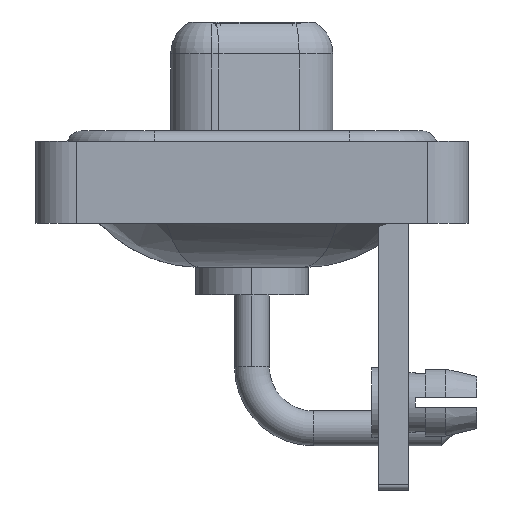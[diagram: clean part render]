
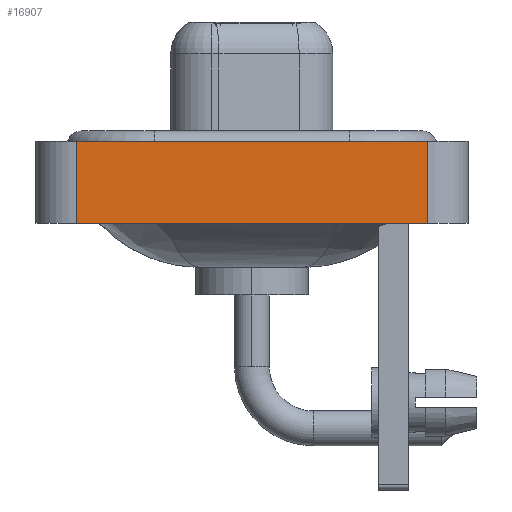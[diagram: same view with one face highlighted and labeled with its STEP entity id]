
A CAD part, left-side view. The second image highlights one B-rep face of the part: STEP entity #16907.
In plain terms, the highlighted planar face has unit normal (-1, 0, 0).
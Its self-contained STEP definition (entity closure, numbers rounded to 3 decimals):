
#25 = EDGE_CURVE ( 'NONE', #10821, #4628, #16702, .T. ) ;
#281 = LINE ( 'NONE', #15452, #17291 ) ;
#883 = VERTEX_POINT ( 'NONE', #17997 ) ;
#1345 = CARTESIAN_POINT ( 'NONE',  ( -7.25, -8.55, -3.6 ) ) ;
#1380 = ORIENTED_EDGE ( 'NONE', *, *, #2059, .F. ) ;
#1501 = CARTESIAN_POINT ( 'NONE',  ( -7.25, -8.55, 0.4 ) ) ;
#1527 = AXIS2_PLACEMENT_3D ( 'NONE', #9806, #12780, #12963 ) ;
#1547 = EDGE_CURVE ( 'NONE', #9805, #10821, #13896, .T. ) ;
#2059 = EDGE_CURVE ( 'NONE', #883, #4628, #7093, .T. ) ;
#2160 = EDGE_LOOP ( 'NONE', ( #3265, #1380, #16736, #16209 ) ) ;
#2559 = CARTESIAN_POINT ( 'NONE',  ( -7.25, -8.55, -3.6 ) ) ;
#3213 = CARTESIAN_POINT ( 'NONE',  ( -7.25, -8.55, 0.4 ) ) ;
#3265 = ORIENTED_EDGE ( 'NONE', *, *, #25, .T. ) ;
#3980 = VECTOR ( 'NONE', #8438, 1000. ) ;
#4022 = CARTESIAN_POINT ( 'NONE',  ( -7.25, -8.55, -3.6 ) ) ;
#4605 = DIRECTION ( 'NONE',  ( 0., -1., 0. ) ) ;
#4628 = VERTEX_POINT ( 'NONE', #1501 ) ;
#5904 = DIRECTION ( 'NONE',  ( 0., 0., 1. ) ) ;
#7093 = LINE ( 'NONE', #3213, #9594 ) ;
#7221 = CARTESIAN_POINT ( 'NONE',  ( -7.25, 8.55, -3.6 ) ) ;
#8438 = DIRECTION ( 'NONE',  ( 0., -1., 0. ) ) ;
#8924 = VECTOR ( 'NONE', #15216, 1000. ) ;
#9594 = VECTOR ( 'NONE', #4605, 1000. ) ;
#9805 = VERTEX_POINT ( 'NONE', #7221 ) ;
#9806 = CARTESIAN_POINT ( 'NONE',  ( -7.25, -8.55, -3.6 ) ) ;
#10821 = VERTEX_POINT ( 'NONE', #1345 ) ;
#12780 = DIRECTION ( 'NONE',  ( -1., 0., 0. ) ) ;
#12963 = DIRECTION ( 'NONE',  ( 0., 0., 1. ) ) ;
#13896 = LINE ( 'NONE', #4022, #3980 ) ;
#13988 = FACE_OUTER_BOUND ( 'NONE', #2160, .T. ) ;
#14525 = EDGE_CURVE ( 'NONE', #9805, #883, #281, .T. ) ;
#15216 = DIRECTION ( 'NONE',  ( 0., 0., 1. ) ) ;
#15452 = CARTESIAN_POINT ( 'NONE',  ( -7.25, 8.55, -3.6 ) ) ;
#16209 = ORIENTED_EDGE ( 'NONE', *, *, #1547, .T. ) ;
#16702 = LINE ( 'NONE', #2559, #8924 ) ;
#16736 = ORIENTED_EDGE ( 'NONE', *, *, #14525, .F. ) ;
#16859 = PLANE ( 'NONE',  #1527 ) ;
#16907 = ADVANCED_FACE ( 'NONE', ( #13988 ), #16859, .T. ) ;
#17291 = VECTOR ( 'NONE', #5904, 1000. ) ;
#17997 = CARTESIAN_POINT ( 'NONE',  ( -7.25, 8.55, 0.4 ) ) ;
